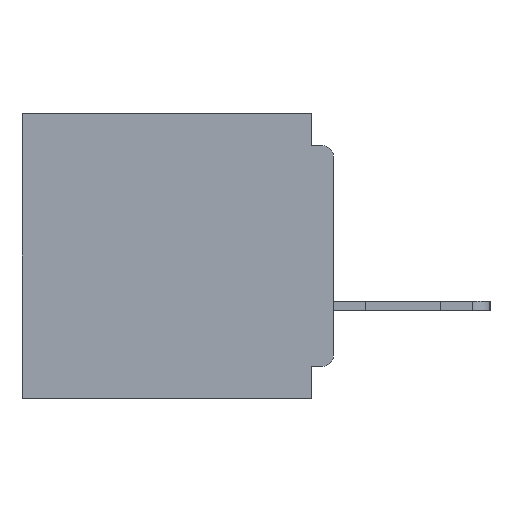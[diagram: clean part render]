
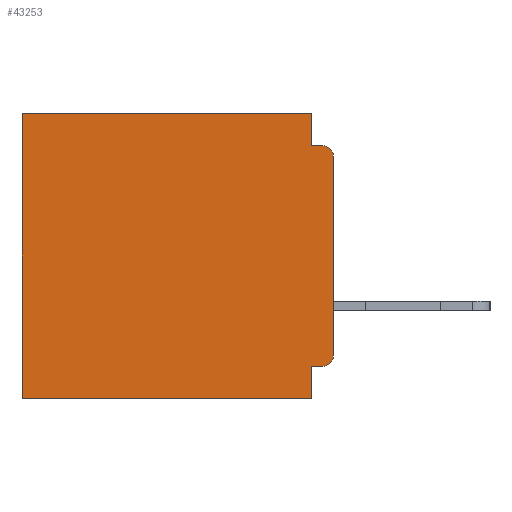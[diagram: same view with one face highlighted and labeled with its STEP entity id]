
A CAD part, left-side view. The second image highlights one B-rep face of the part: STEP entity #43253.
In plain terms, the highlighted planar face has unit normal (-1, 0, 0).
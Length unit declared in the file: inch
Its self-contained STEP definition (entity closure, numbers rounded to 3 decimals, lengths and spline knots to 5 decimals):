
#1404 = CARTESIAN_POINT ( 'NONE',  ( 0.3, 0.031, 0. ) ) ;
#2532 = VERTEX_POINT ( 'NONE', #36893 ) ;
#2896 = ORIENTED_EDGE ( 'NONE', *, *, #6850, .F. ) ;
#2988 = VERTEX_POINT ( 'NONE', #5747 ) ;
#3061 = LINE ( 'NONE', #1404, #41393 ) ;
#3328 = VERTEX_POINT ( 'NONE', #53913 ) ;
#3609 = CARTESIAN_POINT ( 'NONE',  ( 0.3, 0.437, -0.4 ) ) ;
#4510 = CARTESIAN_POINT ( 'NONE',  ( 0.3, 0., -0.045 ) ) ;
#4815 = ORIENTED_EDGE ( 'NONE', *, *, #17192, .F. ) ;
#5747 = CARTESIAN_POINT ( 'NONE',  ( 0.3, 0.031, -0.4 ) ) ;
#6094 = DIRECTION ( 'NONE',  ( 0., 0., -1. ) ) ;
#6531 = LINE ( 'NONE', #34445, #41889 ) ;
#6765 = DIRECTION ( 'NONE',  ( 0., 1., 0. ) ) ;
#6850 = EDGE_CURVE ( 'NONE', #2532, #2988, #55770, .T. ) ;
#7307 = AXIS2_PLACEMENT_3D ( 'NONE', #19172, #51293, #28648 ) ;
#7507 = CARTESIAN_POINT ( 'NONE',  ( 0.3, 0., -0.4 ) ) ;
#7911 = VERTEX_POINT ( 'NONE', #19624 ) ;
#8252 = ORIENTED_EDGE ( 'NONE', *, *, #38419, .F. ) ;
#8302 = EDGE_CURVE ( 'NONE', #26568, #55243, #19468, .T. ) ;
#11771 = LINE ( 'NONE', #27181, #45603 ) ;
#12403 = EDGE_LOOP ( 'NONE', ( #4815, #51520, #29029, #24835, #32664, #31359, #8252, #2896, #35031, #27426 ) ) ;
#13447 = FACE_OUTER_BOUND ( 'NONE', #12403, .T. ) ;
#14445 = CARTESIAN_POINT ( 'NONE',  ( 0.3, 0.031, -0.045 ) ) ;
#14997 = CARTESIAN_POINT ( 'NONE',  ( 0.3, 0.031, -0.4 ) ) ;
#15131 = EDGE_CURVE ( 'NONE', #28617, #26568, #6531, .T. ) ;
#15628 = CARTESIAN_POINT ( 'NONE',  ( 0.3, 0., -0.34 ) ) ;
#17192 = EDGE_CURVE ( 'NONE', #3328, #29839, #35996, .T. ) ;
#17569 = DIRECTION ( 'NONE',  ( 0., 1., 0. ) ) ;
#19172 = CARTESIAN_POINT ( 'NONE',  ( 0.3, 0.015, -0.06 ) ) ;
#19468 = LINE ( 'NONE', #58970, #30307 ) ;
#19624 = CARTESIAN_POINT ( 'NONE',  ( 0.3, 0.015, -0.355 ) ) ;
#20356 = CARTESIAN_POINT ( 'NONE',  ( 0.3, 0., -0.4 ) ) ;
#20701 = CARTESIAN_POINT ( 'NONE',  ( 0.3, 0.031, 0. ) ) ;
#21954 = LINE ( 'NONE', #40508, #34174 ) ;
#24835 = ORIENTED_EDGE ( 'NONE', *, *, #58973, .F. ) ;
#24978 = DIRECTION ( 'NONE',  ( 1., 0., 0. ) ) ;
#26242 = CIRCLE ( 'NONE', #26389, 0.015 ) ;
#26389 = AXIS2_PLACEMENT_3D ( 'NONE', #26452, #58377, #31057 ) ;
#26452 = CARTESIAN_POINT ( 'NONE',  ( 0.3, 0.015, -0.34 ) ) ;
#26568 = VERTEX_POINT ( 'NONE', #50896 ) ;
#27181 = CARTESIAN_POINT ( 'NONE',  ( 0.3, 0., -0.355 ) ) ;
#27426 = ORIENTED_EDGE ( 'NONE', *, *, #37018, .T. ) ;
#28115 = VECTOR ( 'NONE', #35185, 39.37008 ) ;
#28617 = VERTEX_POINT ( 'NONE', #20701 ) ;
#28648 = DIRECTION ( 'NONE',  ( 0., 0., -1. ) ) ;
#29029 = ORIENTED_EDGE ( 'NONE', *, *, #29569, .F. ) ;
#29569 = EDGE_CURVE ( 'NONE', #36013, #32132, #43426, .T. ) ;
#29839 = VERTEX_POINT ( 'NONE', #15628 ) ;
#30307 = VECTOR ( 'NONE', #50108, 39.37008 ) ;
#31057 = DIRECTION ( 'NONE',  ( 0., 0., -1. ) ) ;
#31359 = ORIENTED_EDGE ( 'NONE', *, *, #8302, .T. ) ;
#31760 = DIRECTION ( 'NONE',  ( 0., 1., 0. ) ) ;
#32132 = VERTEX_POINT ( 'NONE', #47361 ) ;
#32664 = ORIENTED_EDGE ( 'NONE', *, *, #15131, .T. ) ;
#34174 = VECTOR ( 'NONE', #17569, 39.37008 ) ;
#34445 = CARTESIAN_POINT ( 'NONE',  ( 0.3, 0., 0. ) ) ;
#35031 = ORIENTED_EDGE ( 'NONE', *, *, #43579, .F. ) ;
#35185 = DIRECTION ( 'NONE',  ( 0., 0., -1. ) ) ;
#35415 = EDGE_CURVE ( 'NONE', #3328, #32132, #36422, .T. ) ;
#35996 = LINE ( 'NONE', #7507, #28115 ) ;
#36013 = VERTEX_POINT ( 'NONE', #14445 ) ;
#36422 = CIRCLE ( 'NONE', #7307, 0.015 ) ;
#36855 = DIRECTION ( 'NONE',  ( 0., -1., 0. ) ) ;
#36893 = CARTESIAN_POINT ( 'NONE',  ( 0.3, 0.031, -0.355 ) ) ;
#37018 = EDGE_CURVE ( 'NONE', #7911, #29839, #26242, .T. ) ;
#38419 = EDGE_CURVE ( 'NONE', #2988, #55243, #21954, .T. ) ;
#40508 = CARTESIAN_POINT ( 'NONE',  ( 0.3, 0., -0.4 ) ) ;
#41393 = VECTOR ( 'NONE', #6094, 39.37008 ) ;
#41889 = VECTOR ( 'NONE', #6765, 39.37008 ) ;
#43253 = ADVANCED_FACE ( 'NONE', ( #13447 ), #47863, .F. ) ;
#43426 = LINE ( 'NONE', #4510, #55527 ) ;
#43579 = EDGE_CURVE ( 'NONE', #7911, #2532, #11771, .T. ) ;
#43678 = VECTOR ( 'NONE', #56280, 39.37008 ) ;
#45603 = VECTOR ( 'NONE', #31760, 39.37008 ) ;
#47361 = CARTESIAN_POINT ( 'NONE',  ( 0.3, 0.015, -0.045 ) ) ;
#47863 = PLANE ( 'NONE',  #50070 ) ;
#50070 = AXIS2_PLACEMENT_3D ( 'NONE', #20356, #24978, #56935 ) ;
#50108 = DIRECTION ( 'NONE',  ( 0., 0., -1. ) ) ;
#50896 = CARTESIAN_POINT ( 'NONE',  ( 0.3, 0.437, 0. ) ) ;
#51293 = DIRECTION ( 'NONE',  ( -1., 0., 0. ) ) ;
#51520 = ORIENTED_EDGE ( 'NONE', *, *, #35415, .T. ) ;
#53913 = CARTESIAN_POINT ( 'NONE',  ( 0.3, 0., -0.06 ) ) ;
#55243 = VERTEX_POINT ( 'NONE', #3609 ) ;
#55527 = VECTOR ( 'NONE', #36855, 39.37008 ) ;
#55770 = LINE ( 'NONE', #14997, #43678 ) ;
#56280 = DIRECTION ( 'NONE',  ( 0., 0., -1. ) ) ;
#56935 = DIRECTION ( 'NONE',  ( 0., 0., -1. ) ) ;
#58377 = DIRECTION ( 'NONE',  ( -1., 0., 0. ) ) ;
#58970 = CARTESIAN_POINT ( 'NONE',  ( 0.3, 0.437, -0.4 ) ) ;
#58973 = EDGE_CURVE ( 'NONE', #28617, #36013, #3061, .T. ) ;
